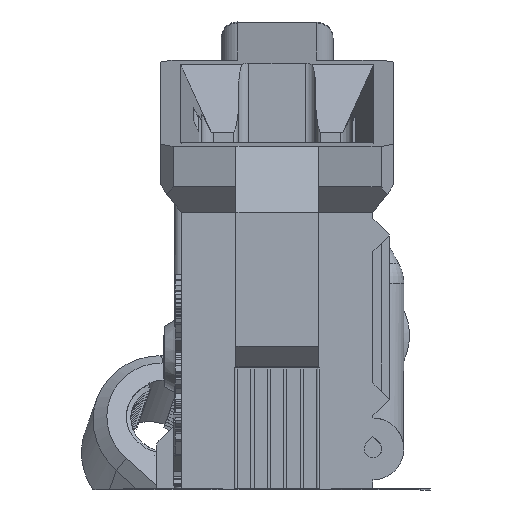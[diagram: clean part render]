
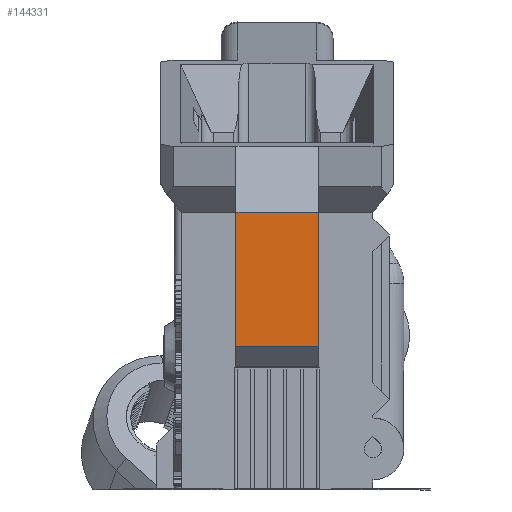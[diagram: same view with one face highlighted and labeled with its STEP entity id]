
A CAD part, left-side view. The second image highlights one B-rep face of the part: STEP entity #144331.
In plain terms, the highlighted planar face has unit normal (-1, 0, 0).
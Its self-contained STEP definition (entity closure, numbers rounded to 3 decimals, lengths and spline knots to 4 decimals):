
#1975 = ORIENTED_EDGE ( 'NONE', *, *, #9023, .F. ) ;
#7855 = DIRECTION ( 'NONE',  ( 0., 1., 0. ) ) ;
#9023 = EDGE_CURVE ( 'NONE', #39536, #70709, #94044, .T. ) ;
#11165 = LINE ( 'NONE', #102464, #109454 ) ;
#31289 = CARTESIAN_POINT ( 'NONE',  ( -4.187, -1.0289, 2.518 ) ) ;
#36492 = DIRECTION ( 'NONE',  ( -1., 0., 0. ) ) ;
#38370 = EDGE_CURVE ( 'NONE', #39536, #95707, #11165, .T. ) ;
#39052 = LINE ( 'NONE', #82838, #61072 ) ;
#39536 = VERTEX_POINT ( 'NONE', #119841 ) ;
#39707 = EDGE_CURVE ( 'NONE', #70709, #146102, #39052, .T. ) ;
#40336 = EDGE_LOOP ( 'NONE', ( #159347, #105937, #164750, #1975 ) ) ;
#45877 = DIRECTION ( 'NONE',  ( 0., 0., 1. ) ) ;
#48688 = LINE ( 'NONE', #31289, #68740 ) ;
#61072 = VECTOR ( 'NONE', #45877, 39.3701 ) ;
#67983 = VECTOR ( 'NONE', #7855, 39.3701 ) ;
#68740 = VECTOR ( 'NONE', #82261, 39.3701 ) ;
#70709 = VERTEX_POINT ( 'NONE', #108460 ) ;
#74018 = DIRECTION ( 'NONE',  ( 0., 1., 0. ) ) ;
#74586 = CARTESIAN_POINT ( 'NONE',  ( -4.187, -1.0289, 1.7032 ) ) ;
#82261 = DIRECTION ( 'NONE',  ( 0., 1., 0. ) ) ;
#82838 = CARTESIAN_POINT ( 'NONE',  ( -4.187, 1.1526, 2.518 ) ) ;
#86815 = CARTESIAN_POINT ( 'NONE',  ( -4.187, 1.1526, 2.518 ) ) ;
#94044 = LINE ( 'NONE', #136291, #67983 ) ;
#95707 = VERTEX_POINT ( 'NONE', #106227 ) ;
#101900 = DIRECTION ( 'NONE',  ( 0., 0., 1. ) ) ;
#102464 = CARTESIAN_POINT ( 'NONE',  ( -4.187, 0.6526, 1.7032 ) ) ;
#105937 = ORIENTED_EDGE ( 'NONE', *, *, #121495, .T. ) ;
#106227 = CARTESIAN_POINT ( 'NONE',  ( -4.187, 0.6526, 2.518 ) ) ;
#108460 = CARTESIAN_POINT ( 'NONE',  ( -4.187, 1.1526, 1.7032 ) ) ;
#109454 = VECTOR ( 'NONE', #101900, 39.3701 ) ;
#119841 = CARTESIAN_POINT ( 'NONE',  ( -4.187, 0.6526, 1.7032 ) ) ;
#121495 = EDGE_CURVE ( 'NONE', #95707, #146102, #48688, .T. ) ;
#136291 = CARTESIAN_POINT ( 'NONE',  ( -4.187, -1.0289, 1.7032 ) ) ;
#144331 = ADVANCED_FACE ( 'NONE', ( #152860 ), #150863, .T. ) ;
#146102 = VERTEX_POINT ( 'NONE', #86815 ) ;
#150195 = AXIS2_PLACEMENT_3D ( 'NONE', #74586, #36492, #74018 ) ;
#150863 = PLANE ( 'NONE',  #150195 ) ;
#152860 = FACE_OUTER_BOUND ( 'NONE', #40336, .T. ) ;
#159347 = ORIENTED_EDGE ( 'NONE', *, *, #38370, .T. ) ;
#164750 = ORIENTED_EDGE ( 'NONE', *, *, #39707, .F. ) ;
